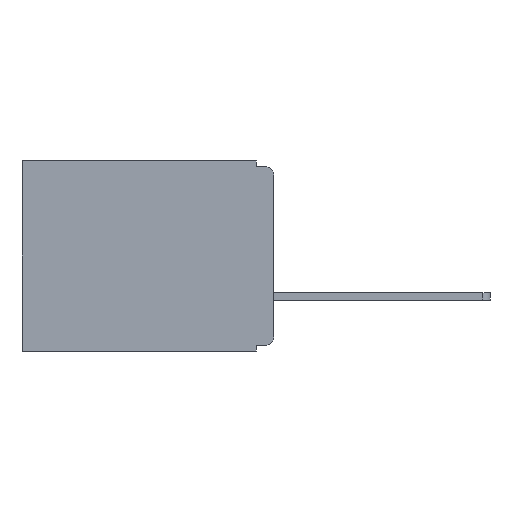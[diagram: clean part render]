
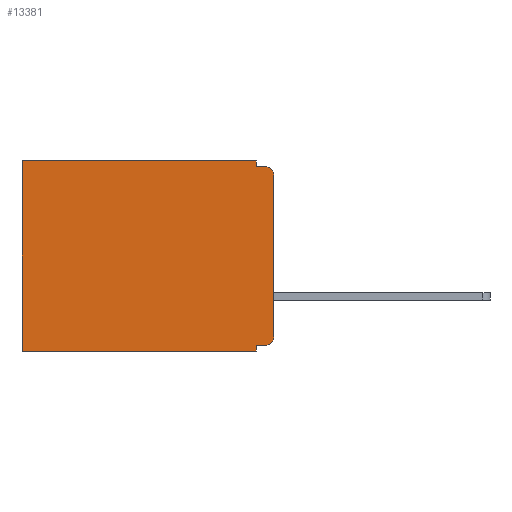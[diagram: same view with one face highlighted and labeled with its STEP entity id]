
A CAD part, left-side view. The second image highlights one B-rep face of the part: STEP entity #13381.
In plain terms, the highlighted planar face has unit normal (-1, 0, 0).
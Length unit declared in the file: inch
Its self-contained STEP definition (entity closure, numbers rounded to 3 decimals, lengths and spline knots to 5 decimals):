
#9 = EDGE_CURVE ( 'NONE', #2697, #5741, #15273, .T. ) ;
#66 = EDGE_CURVE ( 'NONE', #9704, #3239, #13917, .T. ) ;
#1020 = VECTOR ( 'NONE', #16904, 39.37008 ) ;
#1359 = DIRECTION ( 'NONE',  ( 0., -1., 0. ) ) ;
#1509 = VECTOR ( 'NONE', #1359, 39.37008 ) ;
#2435 = ORIENTED_EDGE ( 'NONE', *, *, #13842, .F. ) ;
#2573 = EDGE_CURVE ( 'NONE', #10266, #10361, #11782, .T. ) ;
#2697 = VERTEX_POINT ( 'NONE', #4738 ) ;
#2865 = DIRECTION ( 'NONE',  ( 0., 0., -1. ) ) ;
#3239 = VERTEX_POINT ( 'NONE', #5883 ) ;
#3566 = CARTESIAN_POINT ( 'NONE',  ( 0.3, 0., -0.025 ) ) ;
#3657 = VECTOR ( 'NONE', #16867, 39.37008 ) ;
#3689 = CARTESIAN_POINT ( 'NONE',  ( 0.3, 0., -0.32 ) ) ;
#4030 = ORIENTED_EDGE ( 'NONE', *, *, #5408, .F. ) ;
#4667 = LINE ( 'NONE', #14371, #5108 ) ;
#4738 = CARTESIAN_POINT ( 'NONE',  ( 0.3, 0.437, 0. ) ) ;
#4935 = VECTOR ( 'NONE', #18041, 39.37008 ) ;
#5108 = VECTOR ( 'NONE', #15184, 39.37008 ) ;
#5372 = EDGE_CURVE ( 'NONE', #8046, #7710, #8999, .T. ) ;
#5394 = LINE ( 'NONE', #5713, #1509 ) ;
#5408 = EDGE_CURVE ( 'NONE', #9704, #7710, #4667, .T. ) ;
#5429 = VECTOR ( 'NONE', #14039, 39.37008 ) ;
#5536 = CARTESIAN_POINT ( 'NONE',  ( 0.3, 0.031, -0.33 ) ) ;
#5713 = CARTESIAN_POINT ( 'NONE',  ( 0.3, 0., -0.01 ) ) ;
#5741 = VERTEX_POINT ( 'NONE', #11532 ) ;
#5779 = VECTOR ( 'NONE', #6422, 39.37008 ) ;
#5883 = CARTESIAN_POINT ( 'NONE',  ( 0.3, 0.015, -0.01 ) ) ;
#6121 = AXIS2_PLACEMENT_3D ( 'NONE', #15422, #15439, #2865 ) ;
#6241 = LINE ( 'NONE', #15136, #5779 ) ;
#6293 = ORIENTED_EDGE ( 'NONE', *, *, #5372, .T. ) ;
#6309 = LINE ( 'NONE', #3689, #11086 ) ;
#6422 = DIRECTION ( 'NONE',  ( 0., 0., -1. ) ) ;
#7023 = PLANE ( 'NONE',  #13092 ) ;
#7710 = VERTEX_POINT ( 'NONE', #16435 ) ;
#7900 = ORIENTED_EDGE ( 'NONE', *, *, #66, .T. ) ;
#8046 = VERTEX_POINT ( 'NONE', #9875 ) ;
#8350 = ORIENTED_EDGE ( 'NONE', *, *, #2573, .F. ) ;
#8603 = CARTESIAN_POINT ( 'NONE',  ( 0.3, 0.031, -0.32 ) ) ;
#8800 = ORIENTED_EDGE ( 'NONE', *, *, #9, .T. ) ;
#8999 = CIRCLE ( 'NONE', #14453, 0.015 ) ;
#9615 = CARTESIAN_POINT ( 'NONE',  ( 0.3, 0., 0. ) ) ;
#9704 = VERTEX_POINT ( 'NONE', #3566 ) ;
#9875 = CARTESIAN_POINT ( 'NONE',  ( 0.3, 0.015, -0.32 ) ) ;
#9927 = DIRECTION ( 'NONE',  ( 0., 0., -1. ) ) ;
#10266 = VERTEX_POINT ( 'NONE', #17810 ) ;
#10361 = VERTEX_POINT ( 'NONE', #12248 ) ;
#10685 = VERTEX_POINT ( 'NONE', #8603 ) ;
#11086 = VECTOR ( 'NONE', #13880, 39.37008 ) ;
#11532 = CARTESIAN_POINT ( 'NONE',  ( 0.3, 0.437, -0.33 ) ) ;
#11761 = ORIENTED_EDGE ( 'NONE', *, *, #13469, .F. ) ;
#11782 = LINE ( 'NONE', #17140, #4935 ) ;
#12217 = ORIENTED_EDGE ( 'NONE', *, *, #16370, .T. ) ;
#12248 = CARTESIAN_POINT ( 'NONE',  ( 0.3, 0.031, -0.01 ) ) ;
#12683 = ORIENTED_EDGE ( 'NONE', *, *, #13927, .F. ) ;
#12699 = LINE ( 'NONE', #14000, #1020 ) ;
#12785 = CARTESIAN_POINT ( 'NONE',  ( 0.3, 0.015, -0.305 ) ) ;
#12786 = VERTEX_POINT ( 'NONE', #5536 ) ;
#13092 = AXIS2_PLACEMENT_3D ( 'NONE', #17177, #18577, #9927 ) ;
#13381 = ADVANCED_FACE ( 'NONE', ( #14987 ), #7023, .F. ) ;
#13469 = EDGE_CURVE ( 'NONE', #10361, #3239, #5394, .T. ) ;
#13842 = EDGE_CURVE ( 'NONE', #8046, #10685, #6309, .T. ) ;
#13880 = DIRECTION ( 'NONE',  ( 0., 1., 0. ) ) ;
#13917 = CIRCLE ( 'NONE', #6121, 0.015 ) ;
#13927 = EDGE_CURVE ( 'NONE', #12786, #5741, #12699, .T. ) ;
#14000 = CARTESIAN_POINT ( 'NONE',  ( 0.3, 0., -0.33 ) ) ;
#14039 = DIRECTION ( 'NONE',  ( 0., 1., 0. ) ) ;
#14371 = CARTESIAN_POINT ( 'NONE',  ( 0.3, 0., -0.33 ) ) ;
#14453 = AXIS2_PLACEMENT_3D ( 'NONE', #12785, #17653, #15895 ) ;
#14707 = CARTESIAN_POINT ( 'NONE',  ( 0.3, 0.437, -0.33 ) ) ;
#14987 = FACE_OUTER_BOUND ( 'NONE', #16852, .T. ) ;
#15136 = CARTESIAN_POINT ( 'NONE',  ( 0.3, 0.031, -0.33 ) ) ;
#15184 = DIRECTION ( 'NONE',  ( 0., 0., -1. ) ) ;
#15273 = LINE ( 'NONE', #14707, #3657 ) ;
#15422 = CARTESIAN_POINT ( 'NONE',  ( 0.3, 0.015, -0.025 ) ) ;
#15439 = DIRECTION ( 'NONE',  ( -1., 0., 0. ) ) ;
#15625 = EDGE_CURVE ( 'NONE', #10685, #12786, #6241, .T. ) ;
#15895 = DIRECTION ( 'NONE',  ( 0., 0., -1. ) ) ;
#16370 = EDGE_CURVE ( 'NONE', #10266, #2697, #17067, .T. ) ;
#16435 = CARTESIAN_POINT ( 'NONE',  ( 0.3, 0., -0.305 ) ) ;
#16852 = EDGE_LOOP ( 'NONE', ( #4030, #7900, #11761, #8350, #12217, #8800, #12683, #16994, #2435, #6293 ) ) ;
#16867 = DIRECTION ( 'NONE',  ( 0., 0., -1. ) ) ;
#16904 = DIRECTION ( 'NONE',  ( 0., 1., 0. ) ) ;
#16994 = ORIENTED_EDGE ( 'NONE', *, *, #15625, .F. ) ;
#17067 = LINE ( 'NONE', #9615, #5429 ) ;
#17140 = CARTESIAN_POINT ( 'NONE',  ( 0.3, 0.031, 0. ) ) ;
#17177 = CARTESIAN_POINT ( 'NONE',  ( 0.3, 0., -0.33 ) ) ;
#17653 = DIRECTION ( 'NONE',  ( -1., 0., 0. ) ) ;
#17810 = CARTESIAN_POINT ( 'NONE',  ( 0.3, 0.031, 0. ) ) ;
#18041 = DIRECTION ( 'NONE',  ( 0., 0., -1. ) ) ;
#18577 = DIRECTION ( 'NONE',  ( 1., 0., 0. ) ) ;
